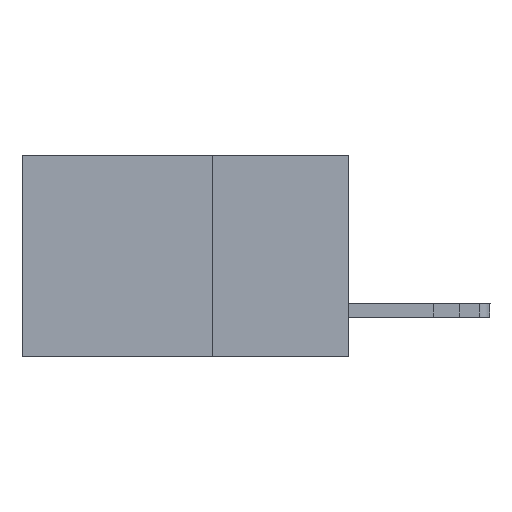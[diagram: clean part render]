
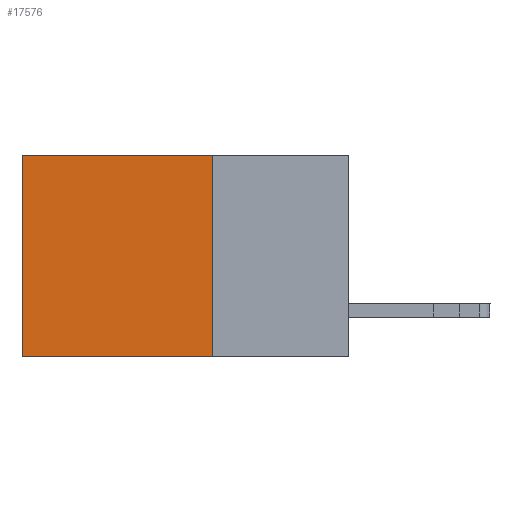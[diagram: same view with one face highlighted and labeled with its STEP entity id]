
A CAD part, left-side view. The second image highlights one B-rep face of the part: STEP entity #17576.
In plain terms, the highlighted planar face has unit normal (-1, 0, 0).
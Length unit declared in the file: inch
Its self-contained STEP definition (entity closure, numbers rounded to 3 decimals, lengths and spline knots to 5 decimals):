
#578 = LINE ( 'NONE', #7843, #10630 ) ;
#593 = CARTESIAN_POINT ( 'NONE',  ( 0.298, 0.25, 0. ) ) ;
#869 = EDGE_CURVE ( 'NONE', #12930, #16697, #8178, .T. ) ;
#1749 = CARTESIAN_POINT ( 'NONE',  ( 0.298, 0.25, 0. ) ) ;
#2850 = CARTESIAN_POINT ( 'NONE',  ( 0.298, 0.6, 0. ) ) ;
#3272 = DIRECTION ( 'NONE',  ( 1., 0., 0. ) ) ;
#3454 = LINE ( 'NONE', #593, #12141 ) ;
#4714 = FACE_OUTER_BOUND ( 'NONE', #12740, .T. ) ;
#4833 = ORIENTED_EDGE ( 'NONE', *, *, #9242, .F. ) ;
#4896 = AXIS2_PLACEMENT_3D ( 'NONE', #1749, #3272, #6152 ) ;
#5127 = EDGE_CURVE ( 'NONE', #15377, #16503, #6646, .T. ) ;
#5427 = VECTOR ( 'NONE', #18656, 39.37008 ) ;
#6152 = DIRECTION ( 'NONE',  ( 0., 0., -1. ) ) ;
#6646 = LINE ( 'NONE', #17221, #5427 ) ;
#7456 = CARTESIAN_POINT ( 'NONE',  ( 0.298, 0.6, -0.37 ) ) ;
#7843 = CARTESIAN_POINT ( 'NONE',  ( 0.298, 0.25, -0.37 ) ) ;
#7938 = DIRECTION ( 'NONE',  ( 0., 1., 0. ) ) ;
#8178 = LINE ( 'NONE', #14905, #12684 ) ;
#8456 = ORIENTED_EDGE ( 'NONE', *, *, #15147, .T. ) ;
#8852 = ORIENTED_EDGE ( 'NONE', *, *, #869, .T. ) ;
#9242 = EDGE_CURVE ( 'NONE', #16503, #16697, #578, .T. ) ;
#10630 = VECTOR ( 'NONE', #7938, 39.37008 ) ;
#10889 = DIRECTION ( 'NONE',  ( 0., 1., 0. ) ) ;
#12141 = VECTOR ( 'NONE', #10889, 39.37008 ) ;
#12684 = VECTOR ( 'NONE', #16330, 39.37008 ) ;
#12740 = EDGE_LOOP ( 'NONE', ( #8852, #4833, #18321, #8456 ) ) ;
#12930 = VERTEX_POINT ( 'NONE', #2850 ) ;
#14520 = CARTESIAN_POINT ( 'NONE',  ( 0.298, 0.25, -0.37 ) ) ;
#14801 = CARTESIAN_POINT ( 'NONE',  ( 0.298, 0.25, 0. ) ) ;
#14905 = CARTESIAN_POINT ( 'NONE',  ( 0.298, 0.6, 0. ) ) ;
#15147 = EDGE_CURVE ( 'NONE', #15377, #12930, #3454, .T. ) ;
#15377 = VERTEX_POINT ( 'NONE', #14801 ) ;
#16330 = DIRECTION ( 'NONE',  ( 0., 0., -1. ) ) ;
#16503 = VERTEX_POINT ( 'NONE', #14520 ) ;
#16541 = PLANE ( 'NONE',  #4896 ) ;
#16697 = VERTEX_POINT ( 'NONE', #7456 ) ;
#17221 = CARTESIAN_POINT ( 'NONE',  ( 0.298, 0.25, 0. ) ) ;
#17576 = ADVANCED_FACE ( 'NONE', ( #4714 ), #16541, .F. ) ;
#18321 = ORIENTED_EDGE ( 'NONE', *, *, #5127, .F. ) ;
#18656 = DIRECTION ( 'NONE',  ( 0., 0., -1. ) ) ;
